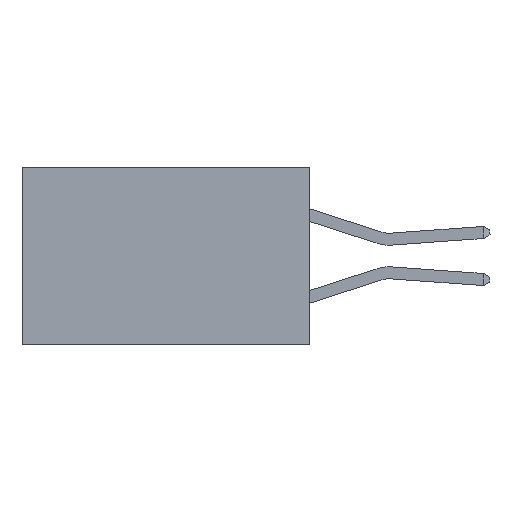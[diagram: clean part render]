
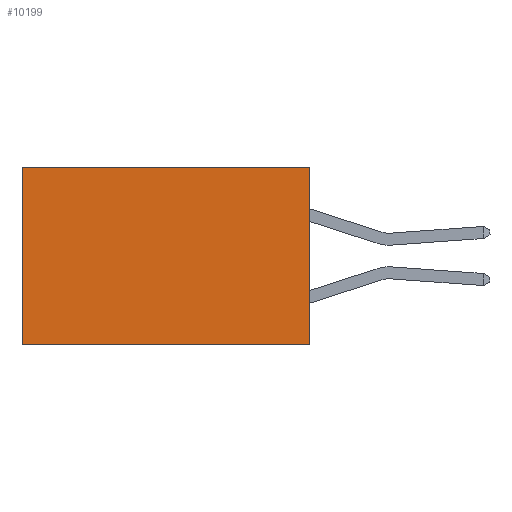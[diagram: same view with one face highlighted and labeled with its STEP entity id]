
A CAD part, left-side view. The second image highlights one B-rep face of the part: STEP entity #10199.
In plain terms, the highlighted planar face has unit normal (-1, 0, 0).
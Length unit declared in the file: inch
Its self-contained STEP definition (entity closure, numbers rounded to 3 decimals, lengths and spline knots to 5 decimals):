
#92 = CARTESIAN_POINT ( 'NONE',  ( 0.298, 0., -0.37 ) ) ;
#125 = ORIENTED_EDGE ( 'NONE', *, *, #6091, .T. ) ;
#522 = CARTESIAN_POINT ( 'NONE',  ( 0.298, 0., 0. ) ) ;
#1383 = DIRECTION ( 'NONE',  ( 0., 0., -1. ) ) ;
#1636 = VERTEX_POINT ( 'NONE', #9970 ) ;
#1973 = ORIENTED_EDGE ( 'NONE', *, *, #5976, .T. ) ;
#2423 = LINE ( 'NONE', #5813, #4451 ) ;
#2554 = CARTESIAN_POINT ( 'NONE',  ( 0.298, 0.6, 0. ) ) ;
#2633 = DIRECTION ( 'NONE',  ( 0., 1., 0. ) ) ;
#2962 = PLANE ( 'NONE',  #8107 ) ;
#3012 = VERTEX_POINT ( 'NONE', #9707 ) ;
#3256 = CARTESIAN_POINT ( 'NONE',  ( 0.298, 0., -0.37 ) ) ;
#3360 = DIRECTION ( 'NONE',  ( 0., 1., 0. ) ) ;
#3901 = EDGE_CURVE ( 'NONE', #1636, #7407, #5163, .T. ) ;
#4073 = EDGE_CURVE ( 'NONE', #7407, #3012, #9850, .T. ) ;
#4451 = VECTOR ( 'NONE', #9220, 39.37008 ) ;
#4673 = ORIENTED_EDGE ( 'NONE', *, *, #3901, .F. ) ;
#5163 = LINE ( 'NONE', #10970, #7173 ) ;
#5447 = EDGE_LOOP ( 'NONE', ( #1973, #9116, #4673, #125 ) ) ;
#5813 = CARTESIAN_POINT ( 'NONE',  ( 0.298, 0.6, 0. ) ) ;
#5854 = DIRECTION ( 'NONE',  ( 0., 0., -1. ) ) ;
#5976 = EDGE_CURVE ( 'NONE', #9817, #3012, #2423, .T. ) ;
#6091 = EDGE_CURVE ( 'NONE', #1636, #9817, #8194, .T. ) ;
#6500 = DIRECTION ( 'NONE',  ( 1., 0., 0. ) ) ;
#7173 = VECTOR ( 'NONE', #5854, 39.37008 ) ;
#7407 = VERTEX_POINT ( 'NONE', #3256 ) ;
#7567 = VECTOR ( 'NONE', #2633, 39.37008 ) ;
#8107 = AXIS2_PLACEMENT_3D ( 'NONE', #522, #6500, #1383 ) ;
#8194 = LINE ( 'NONE', #10222, #10208 ) ;
#9116 = ORIENTED_EDGE ( 'NONE', *, *, #4073, .F. ) ;
#9220 = DIRECTION ( 'NONE',  ( 0., 0., -1. ) ) ;
#9707 = CARTESIAN_POINT ( 'NONE',  ( 0.298, 0.6, -0.37 ) ) ;
#9817 = VERTEX_POINT ( 'NONE', #2554 ) ;
#9850 = LINE ( 'NONE', #92, #7567 ) ;
#9970 = CARTESIAN_POINT ( 'NONE',  ( 0.298, 0., 0. ) ) ;
#10199 = ADVANCED_FACE ( 'NONE', ( #10242 ), #2962, .F. ) ;
#10208 = VECTOR ( 'NONE', #3360, 39.37008 ) ;
#10222 = CARTESIAN_POINT ( 'NONE',  ( 0.298, 0., 0. ) ) ;
#10242 = FACE_OUTER_BOUND ( 'NONE', #5447, .T. ) ;
#10970 = CARTESIAN_POINT ( 'NONE',  ( 0.298, 0., 0. ) ) ;
